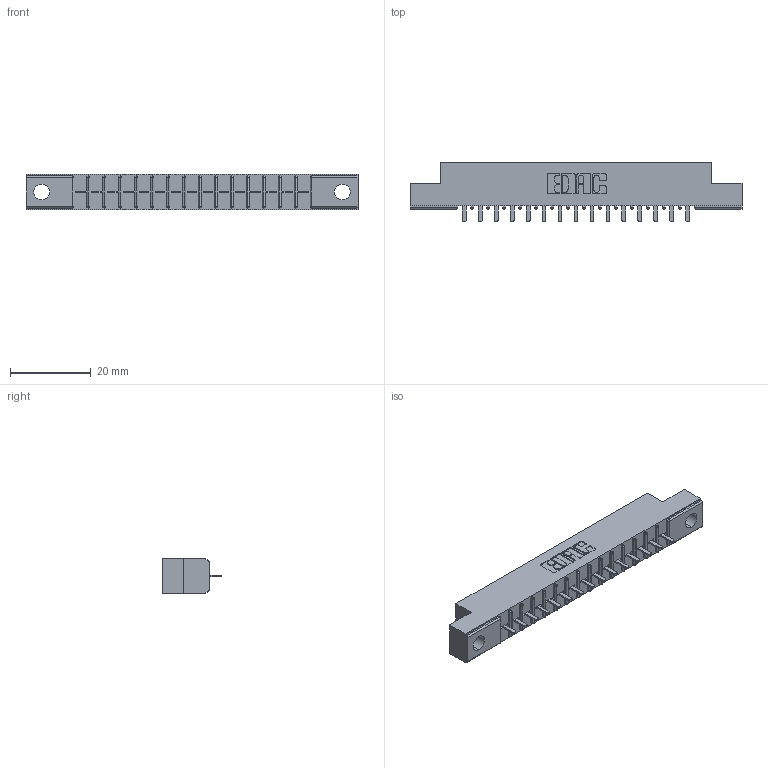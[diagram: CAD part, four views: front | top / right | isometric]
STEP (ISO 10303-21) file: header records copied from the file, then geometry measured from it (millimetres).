
FILE_DESCRIPTION (( 'STEP AP203' ), '1' );
FILE_NAME ('316-015-421-104.STEP', '2020-09-22T17:29:04', ( '' ), ( '' ), 'SwSTEP 2.0', 'SolidWorks 2020', '' );
FILE_SCHEMA (( 'CONFIG_CONTROL_DESIGN' ));
Length unit declared in the file: inch
Products named in the file (3): 306-290-001_121; 316-015-421-104; 306 Part_.156 Dia
Assembly tree (16 placements, depth 2):
  316-015-421-104
    306 Part_.156 Dia
    306-290-001_121  x15
Bounding box: 82.45 x 14.88 x 8.71 mm (x, y, z)
Volume: 5486.7 mm3; surface area: 7640.9 mm2
Topology: 16 solids, 16 shells, 1180 faces, 3307 edges, 2122 vertices
Faces by surface type: plane 787, cylinder 333, sphere 60
Entity records: 17860 total; most frequent: CARTESIAN_POINT 2998, ORIENTED_EDGE 2966, DIRECTION 2951, EDGE_CURVE 1483, LINE 1153, VECTOR 1153, VERTEX_POINT 946, AXIS2_PLACEMENT_3D 899
